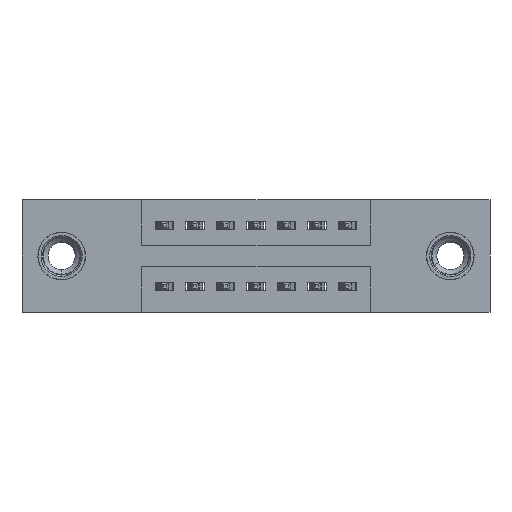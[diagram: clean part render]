
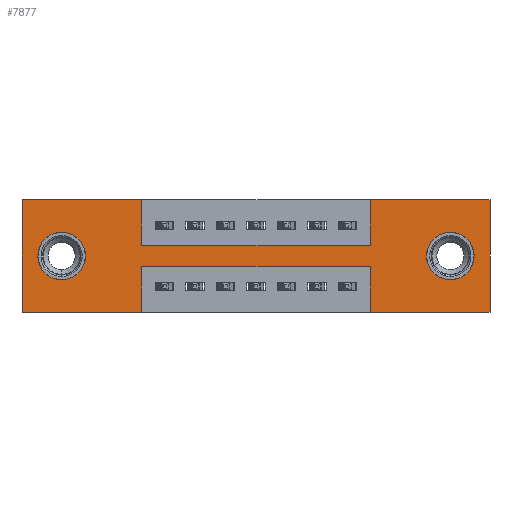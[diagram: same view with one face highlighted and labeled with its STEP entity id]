
A CAD part, front view. The second image highlights one B-rep face of the part: STEP entity #7877.
In plain terms, the highlighted planar face has unit normal (0, -1, 0).
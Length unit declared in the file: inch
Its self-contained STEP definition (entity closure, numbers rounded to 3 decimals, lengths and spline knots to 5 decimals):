
#209 = DIRECTION ( 'NONE',  ( 0., 0., -1. ) ) ;
#260 = ORIENTED_EDGE ( 'NONE', *, *, #10524, .F. ) ;
#261 = ORIENTED_EDGE ( 'NONE', *, *, #7609, .F. ) ;
#296 = CIRCLE ( 'NONE', #1766, 0.078 ) ;
#343 = EDGE_CURVE ( 'NONE', #4326, #10235, #10113, .T. ) ;
#355 = AXIS2_PLACEMENT_3D ( 'NONE', #2334, #4160, #6801 ) ;
#690 = CARTESIAN_POINT ( 'NONE',  ( 0.13, 0., -0.107 ) ) ;
#711 = CARTESIAN_POINT ( 'NONE',  ( 0.3925, 0., -0.22 ) ) ;
#860 = CARTESIAN_POINT ( 'NONE',  ( 0., 0., 0. ) ) ;
#910 = ORIENTED_EDGE ( 'NONE', *, *, #7278, .F. ) ;
#936 = VERTEX_POINT ( 'NONE', #5385 ) ;
#1024 = LINE ( 'NONE', #8199, #6069 ) ;
#1179 = DIRECTION ( 'NONE',  ( 0., 0., -1. ) ) ;
#1204 = CARTESIAN_POINT ( 'NONE',  ( 0., 0., -0.37 ) ) ;
#1212 = LINE ( 'NONE', #10092, #2568 ) ;
#1550 = VECTOR ( 'NONE', #5149, 39.37008 ) ;
#1645 = LINE ( 'NONE', #6267, #3943 ) ;
#1685 = DIRECTION ( 'NONE',  ( -1., 0., 0. ) ) ;
#1687 = ORIENTED_EDGE ( 'NONE', *, *, #7644, .F. ) ;
#1766 = AXIS2_PLACEMENT_3D ( 'NONE', #6440, #2054, #2091 ) ;
#1882 = CARTESIAN_POINT ( 'NONE',  ( 0.3925, 0., -0.37 ) ) ;
#1995 = ORIENTED_EDGE ( 'NONE', *, *, #8887, .F. ) ;
#2054 = DIRECTION ( 'NONE',  ( 0., 1., 0. ) ) ;
#2091 = DIRECTION ( 'NONE',  ( 0., 0., 1. ) ) ;
#2261 = ORIENTED_EDGE ( 'NONE', *, *, #4934, .F. ) ;
#2333 = LINE ( 'NONE', #7928, #1550 ) ;
#2334 = CARTESIAN_POINT ( 'NONE',  ( 1.405, 0., -0.185 ) ) ;
#2336 = VERTEX_POINT ( 'NONE', #8342 ) ;
#2430 = EDGE_LOOP ( 'NONE', ( #10405, #5566 ) ) ;
#2521 = EDGE_CURVE ( 'NONE', #5019, #6939, #3582, .T. ) ;
#2568 = VECTOR ( 'NONE', #5686, 39.37008 ) ;
#2625 = LINE ( 'NONE', #3432, #6314 ) ;
#2678 = DIRECTION ( 'NONE',  ( 0., 0., 1. ) ) ;
#2822 = CARTESIAN_POINT ( 'NONE',  ( 1.1425, 0., -0.37 ) ) ;
#3076 = CARTESIAN_POINT ( 'NONE',  ( 0., 0., -0.37 ) ) ;
#3107 = VECTOR ( 'NONE', #2678, 39.37008 ) ;
#3229 = ORIENTED_EDGE ( 'NONE', *, *, #4668, .F. ) ;
#3339 = VERTEX_POINT ( 'NONE', #6839 ) ;
#3364 = EDGE_CURVE ( 'NONE', #6504, #7553, #6189, .T. ) ;
#3376 = LINE ( 'NONE', #1882, #8454 ) ;
#3432 = CARTESIAN_POINT ( 'NONE',  ( 0., 0., 0. ) ) ;
#3451 = CARTESIAN_POINT ( 'NONE',  ( 1.535, 0., 0. ) ) ;
#3582 = LINE ( 'NONE', #3076, #4982 ) ;
#3625 = VECTOR ( 'NONE', #8859, 39.37008 ) ;
#3638 = LINE ( 'NONE', #711, #3625 ) ;
#3776 = CARTESIAN_POINT ( 'NONE',  ( 0.3925, 0., -0.22 ) ) ;
#3943 = VECTOR ( 'NONE', #7190, 39.37008 ) ;
#3993 = ORIENTED_EDGE ( 'NONE', *, *, #4652, .F. ) ;
#4067 = VERTEX_POINT ( 'NONE', #9557 ) ;
#4160 = DIRECTION ( 'NONE',  ( 0., 1., 0. ) ) ;
#4173 = DIRECTION ( 'NONE',  ( 0., 1., 0. ) ) ;
#4241 = CARTESIAN_POINT ( 'NONE',  ( 0.3925, 0., -0.15 ) ) ;
#4264 = EDGE_CURVE ( 'NONE', #10235, #4326, #296, .T. ) ;
#4326 = VERTEX_POINT ( 'NONE', #10868 ) ;
#4330 = DIRECTION ( 'NONE',  ( 1., 0., 0. ) ) ;
#4652 = EDGE_CURVE ( 'NONE', #936, #10351, #5336, .T. ) ;
#4668 = EDGE_CURVE ( 'NONE', #3339, #936, #2333, .T. ) ;
#4864 = EDGE_LOOP ( 'NONE', ( #1995, #10960, #2261, #8973, #260, #3993, #3229, #261, #7906, #11083, #1687, #910 ) ) ;
#4934 = EDGE_CURVE ( 'NONE', #6939, #2336, #8491, .T. ) ;
#4935 = VECTOR ( 'NONE', #7763, 39.37008 ) ;
#4982 = VECTOR ( 'NONE', #1685, 39.37008 ) ;
#5019 = VERTEX_POINT ( 'NONE', #6894 ) ;
#5149 = DIRECTION ( 'NONE',  ( 0., 0., 1. ) ) ;
#5169 = LINE ( 'NONE', #4241, #8888 ) ;
#5336 = LINE ( 'NONE', #7815, #7937 ) ;
#5385 = CARTESIAN_POINT ( 'NONE',  ( 1.1425, 0., 0. ) ) ;
#5566 = ORIENTED_EDGE ( 'NONE', *, *, #11356, .T. ) ;
#5568 = CARTESIAN_POINT ( 'NONE',  ( 1.1425, 0., -0.37 ) ) ;
#5686 = DIRECTION ( 'NONE',  ( 0., 0., -1. ) ) ;
#5747 = EDGE_CURVE ( 'NONE', #5757, #8596, #2625, .T. ) ;
#5757 = VERTEX_POINT ( 'NONE', #11032 ) ;
#5933 = DIRECTION ( 'NONE',  ( 1., 0., 0. ) ) ;
#6069 = VECTOR ( 'NONE', #1179, 39.37008 ) ;
#6151 = CARTESIAN_POINT ( 'NONE',  ( 0.3925, 0., 0. ) ) ;
#6189 = CIRCLE ( 'NONE', #355, 0.078 ) ;
#6226 = CARTESIAN_POINT ( 'NONE',  ( 0., 0., -0.37 ) ) ;
#6267 = CARTESIAN_POINT ( 'NONE',  ( 0., 0., -0.37 ) ) ;
#6314 = VECTOR ( 'NONE', #6999, 39.37008 ) ;
#6410 = PLANE ( 'NONE',  #6537 ) ;
#6440 = CARTESIAN_POINT ( 'NONE',  ( 0.13, 0., -0.185 ) ) ;
#6474 = EDGE_CURVE ( 'NONE', #8596, #4067, #1212, .T. ) ;
#6504 = VERTEX_POINT ( 'NONE', #6589 ) ;
#6537 = AXIS2_PLACEMENT_3D ( 'NONE', #1204, #9021, #7306 ) ;
#6589 = CARTESIAN_POINT ( 'NONE',  ( 1.405, 0., -0.107 ) ) ;
#6764 = CARTESIAN_POINT ( 'NONE',  ( 1.405, 0., -0.263 ) ) ;
#6801 = DIRECTION ( 'NONE',  ( 0., 0., -1. ) ) ;
#6839 = CARTESIAN_POINT ( 'NONE',  ( 1.1425, 0., -0.15 ) ) ;
#6894 = CARTESIAN_POINT ( 'NONE',  ( 1.535, 0., -0.37 ) ) ;
#6939 = VERTEX_POINT ( 'NONE', #5568 ) ;
#6999 = DIRECTION ( 'NONE',  ( 1., 0., 0. ) ) ;
#7083 = AXIS2_PLACEMENT_3D ( 'NONE', #7678, #8583, #7641 ) ;
#7190 = DIRECTION ( 'NONE',  ( -1., 0., 0. ) ) ;
#7237 = VERTEX_POINT ( 'NONE', #3776 ) ;
#7257 = VERTEX_POINT ( 'NONE', #6226 ) ;
#7278 = EDGE_CURVE ( 'NONE', #7466, #7257, #1645, .T. ) ;
#7306 = DIRECTION ( 'NONE',  ( 0., 0., -1. ) ) ;
#7466 = VERTEX_POINT ( 'NONE', #8509 ) ;
#7553 = VERTEX_POINT ( 'NONE', #6764 ) ;
#7609 = EDGE_CURVE ( 'NONE', #4067, #3339, #5169, .T. ) ;
#7626 = DIRECTION ( 'NONE',  ( 0., 0., 1. ) ) ;
#7641 = DIRECTION ( 'NONE',  ( 0., 0., -1. ) ) ;
#7644 = EDGE_CURVE ( 'NONE', #7257, #5757, #11011, .T. ) ;
#7678 = CARTESIAN_POINT ( 'NONE',  ( 1.405, 0., -0.185 ) ) ;
#7763 = DIRECTION ( 'NONE',  ( 0., 0., 1. ) ) ;
#7815 = CARTESIAN_POINT ( 'NONE',  ( 0., 0., 0. ) ) ;
#7877 = ADVANCED_FACE ( 'NONE', ( #10003, #9449, #8877 ), #6410, .T. ) ;
#7906 = ORIENTED_EDGE ( 'NONE', *, *, #6474, .F. ) ;
#7909 = ORIENTED_EDGE ( 'NONE', *, *, #343, .T. ) ;
#7928 = CARTESIAN_POINT ( 'NONE',  ( 1.1425, 0., 0. ) ) ;
#7937 = VECTOR ( 'NONE', #4330, 39.37008 ) ;
#8199 = CARTESIAN_POINT ( 'NONE',  ( 1.535, 0., 0. ) ) ;
#8342 = CARTESIAN_POINT ( 'NONE',  ( 1.1425, 0., -0.22 ) ) ;
#8454 = VECTOR ( 'NONE', #209, 39.37008 ) ;
#8491 = LINE ( 'NONE', #2822, #4935 ) ;
#8509 = CARTESIAN_POINT ( 'NONE',  ( 0.3925, 0., -0.37 ) ) ;
#8577 = EDGE_CURVE ( 'NONE', #2336, #7237, #3638, .T. ) ;
#8583 = DIRECTION ( 'NONE',  ( 0., 1., 0. ) ) ;
#8596 = VERTEX_POINT ( 'NONE', #6151 ) ;
#8859 = DIRECTION ( 'NONE',  ( -1., 0., 0. ) ) ;
#8877 = FACE_OUTER_BOUND ( 'NONE', #4864, .T. ) ;
#8887 = EDGE_CURVE ( 'NONE', #7237, #7466, #3376, .T. ) ;
#8888 = VECTOR ( 'NONE', #5933, 39.37008 ) ;
#8973 = ORIENTED_EDGE ( 'NONE', *, *, #2521, .F. ) ;
#9021 = DIRECTION ( 'NONE',  ( 0., -1., 0. ) ) ;
#9449 = FACE_BOUND ( 'NONE', #10393, .T. ) ;
#9535 = AXIS2_PLACEMENT_3D ( 'NONE', #9542, #4173, #7626 ) ;
#9542 = CARTESIAN_POINT ( 'NONE',  ( 0.13, 0., -0.185 ) ) ;
#9557 = CARTESIAN_POINT ( 'NONE',  ( 0.3925, 0., -0.15 ) ) ;
#10003 = FACE_BOUND ( 'NONE', #2430, .T. ) ;
#10092 = CARTESIAN_POINT ( 'NONE',  ( 0.3925, 0., 0. ) ) ;
#10113 = CIRCLE ( 'NONE', #9535, 0.078 ) ;
#10235 = VERTEX_POINT ( 'NONE', #690 ) ;
#10351 = VERTEX_POINT ( 'NONE', #3451 ) ;
#10393 = EDGE_LOOP ( 'NONE', ( #11218, #7909 ) ) ;
#10405 = ORIENTED_EDGE ( 'NONE', *, *, #3364, .T. ) ;
#10524 = EDGE_CURVE ( 'NONE', #10351, #5019, #1024, .T. ) ;
#10868 = CARTESIAN_POINT ( 'NONE',  ( 0.13, 0., -0.263 ) ) ;
#10960 = ORIENTED_EDGE ( 'NONE', *, *, #8577, .F. ) ;
#11011 = LINE ( 'NONE', #860, #3107 ) ;
#11032 = CARTESIAN_POINT ( 'NONE',  ( 0., 0., 0. ) ) ;
#11083 = ORIENTED_EDGE ( 'NONE', *, *, #5747, .F. ) ;
#11209 = CIRCLE ( 'NONE', #7083, 0.078 ) ;
#11218 = ORIENTED_EDGE ( 'NONE', *, *, #4264, .T. ) ;
#11356 = EDGE_CURVE ( 'NONE', #7553, #6504, #11209, .T. ) ;
